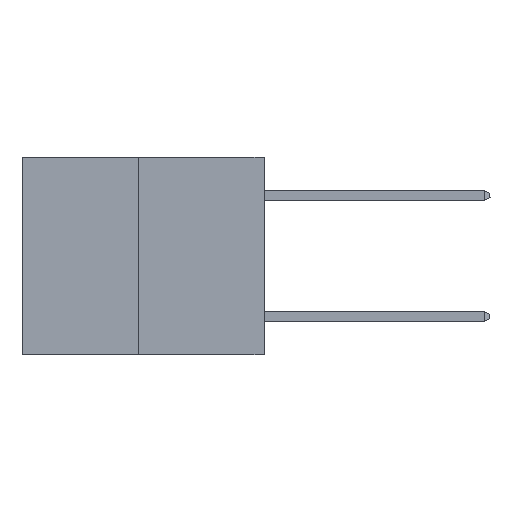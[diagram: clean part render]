
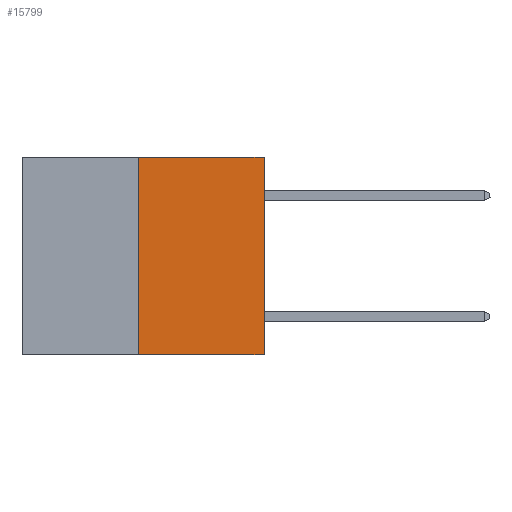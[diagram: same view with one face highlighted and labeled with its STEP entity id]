
A CAD part, left-side view. The second image highlights one B-rep face of the part: STEP entity #15799.
In plain terms, the highlighted planar face has unit normal (-1, 0, 0).
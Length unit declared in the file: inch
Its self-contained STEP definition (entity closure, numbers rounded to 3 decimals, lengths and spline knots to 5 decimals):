
#823 = VERTEX_POINT ( 'NONE', #14452 ) ;
#972 = CARTESIAN_POINT ( 'NONE',  ( 0., 0., -0.49 ) ) ;
#1129 = CARTESIAN_POINT ( 'NONE',  ( 0., 0.6, 0. ) ) ;
#2145 = VECTOR ( 'NONE', #8690, 39.37008 ) ;
#3264 = CARTESIAN_POINT ( 'NONE',  ( 0., 0.6, -0.49 ) ) ;
#4665 = CARTESIAN_POINT ( 'NONE',  ( 0., 0.312, -0.49 ) ) ;
#4994 = PLANE ( 'NONE',  #11545 ) ;
#5222 = EDGE_CURVE ( 'NONE', #14399, #823, #13875, .T. ) ;
#6642 = LINE ( 'NONE', #3264, #2145 ) ;
#6920 = DIRECTION ( 'NONE',  ( 0., 0., -1. ) ) ;
#7289 = CARTESIAN_POINT ( 'NONE',  ( 0., 0.6, 0. ) ) ;
#7609 = EDGE_CURVE ( 'NONE', #13280, #823, #23848, .T. ) ;
#8149 = DIRECTION ( 'NONE',  ( 0., 0., 1. ) ) ;
#8690 = DIRECTION ( 'NONE',  ( 0., -1., 0. ) ) ;
#8714 = CARTESIAN_POINT ( 'NONE',  ( 0., 0.312, 0. ) ) ;
#8962 = EDGE_CURVE ( 'NONE', #22332, #13280, #6642, .T. ) ;
#9469 = VECTOR ( 'NONE', #11454, 39.37008 ) ;
#11454 = DIRECTION ( 'NONE',  ( 0., -1., 0. ) ) ;
#11545 = AXIS2_PLACEMENT_3D ( 'NONE', #1129, #16342, #6920 ) ;
#11865 = ORIENTED_EDGE ( 'NONE', *, *, #5222, .F. ) ;
#12953 = LINE ( 'NONE', #19643, #20955 ) ;
#12986 = ORIENTED_EDGE ( 'NONE', *, *, #7609, .T. ) ;
#13280 = VERTEX_POINT ( 'NONE', #972 ) ;
#13472 = EDGE_CURVE ( 'NONE', #22332, #14399, #12953, .T. ) ;
#13875 = LINE ( 'NONE', #7289, #9469 ) ;
#14399 = VERTEX_POINT ( 'NONE', #8714 ) ;
#14452 = CARTESIAN_POINT ( 'NONE',  ( 0., 0., 0. ) ) ;
#15072 = ORIENTED_EDGE ( 'NONE', *, *, #13472, .F. ) ;
#15799 = ADVANCED_FACE ( 'NONE', ( #21648 ), #4994, .F. ) ;
#16131 = ORIENTED_EDGE ( 'NONE', *, *, #8962, .T. ) ;
#16342 = DIRECTION ( 'NONE',  ( 1., 0., 0. ) ) ;
#19643 = CARTESIAN_POINT ( 'NONE',  ( 0., 0.312, -0.49 ) ) ;
#19914 = DIRECTION ( 'NONE',  ( 0., 0., 1. ) ) ;
#20053 = EDGE_LOOP ( 'NONE', ( #15072, #16131, #12986, #11865 ) ) ;
#20274 = VECTOR ( 'NONE', #8149, 39.37008 ) ;
#20955 = VECTOR ( 'NONE', #19914, 39.37008 ) ;
#21405 = CARTESIAN_POINT ( 'NONE',  ( 0., 0., 0. ) ) ;
#21648 = FACE_OUTER_BOUND ( 'NONE', #20053, .T. ) ;
#22332 = VERTEX_POINT ( 'NONE', #4665 ) ;
#23848 = LINE ( 'NONE', #21405, #20274 ) ;
